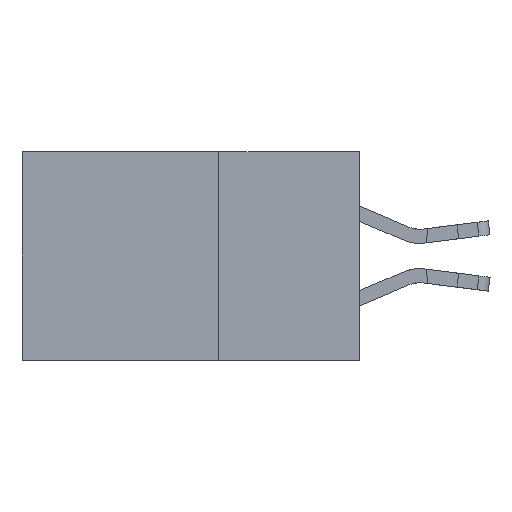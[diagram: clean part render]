
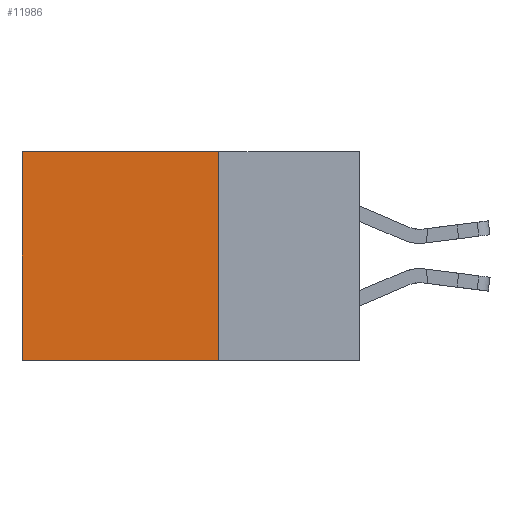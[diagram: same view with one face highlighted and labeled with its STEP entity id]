
A CAD part, left-side view. The second image highlights one B-rep face of the part: STEP entity #11986.
In plain terms, the highlighted planar face has unit normal (-1, 0, 0).
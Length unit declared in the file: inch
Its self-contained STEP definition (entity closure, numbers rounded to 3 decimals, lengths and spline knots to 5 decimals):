
#1357 = CARTESIAN_POINT ( 'NONE',  ( 0.2875, 0.6, 0. ) ) ;
#1444 = AXIS2_PLACEMENT_3D ( 'NONE', #11894, #2779, #13397 ) ;
#1705 = EDGE_CURVE ( 'NONE', #4760, #7678, #9767, .T. ) ;
#1989 = VECTOR ( 'NONE', #11844, 39.37008 ) ;
#2409 = ORIENTED_EDGE ( 'NONE', *, *, #8703, .F. ) ;
#2779 = DIRECTION ( 'NONE',  ( 1., 0., 0. ) ) ;
#3155 = CARTESIAN_POINT ( 'NONE',  ( 0.2875, 0.25, 0. ) ) ;
#3195 = VERTEX_POINT ( 'NONE', #11179 ) ;
#3923 = VECTOR ( 'NONE', #14336, 39.37008 ) ;
#4669 = VECTOR ( 'NONE', #4840, 39.37008 ) ;
#4675 = EDGE_CURVE ( 'NONE', #18759, #3195, #18023, .T. ) ;
#4760 = VERTEX_POINT ( 'NONE', #9041 ) ;
#4840 = DIRECTION ( 'NONE',  ( 0., 1., 0. ) ) ;
#6440 = CARTESIAN_POINT ( 'NONE',  ( 0.2875, 0.25, -0.37 ) ) ;
#6936 = ORIENTED_EDGE ( 'NONE', *, *, #4675, .F. ) ;
#7443 = ORIENTED_EDGE ( 'NONE', *, *, #10565, .T. ) ;
#7678 = VERTEX_POINT ( 'NONE', #17690 ) ;
#8703 = EDGE_CURVE ( 'NONE', #3195, #7678, #8784, .T. ) ;
#8784 = LINE ( 'NONE', #6440, #4669 ) ;
#9041 = CARTESIAN_POINT ( 'NONE',  ( 0.2875, 0.6, 0. ) ) ;
#9308 = VECTOR ( 'NONE', #10592, 39.37008 ) ;
#9767 = LINE ( 'NONE', #1357, #9308 ) ;
#10351 = CARTESIAN_POINT ( 'NONE',  ( 0.2875, 0.25, 0. ) ) ;
#10565 = EDGE_CURVE ( 'NONE', #18759, #4760, #15951, .T. ) ;
#10592 = DIRECTION ( 'NONE',  ( 0., 0., -1. ) ) ;
#11179 = CARTESIAN_POINT ( 'NONE',  ( 0.2875, 0.25, -0.37 ) ) ;
#11844 = DIRECTION ( 'NONE',  ( 0., 0., -1. ) ) ;
#11894 = CARTESIAN_POINT ( 'NONE',  ( 0.2875, 0.25, 0. ) ) ;
#11986 = ADVANCED_FACE ( 'NONE', ( #15643 ), #19264, .F. ) ;
#13397 = DIRECTION ( 'NONE',  ( 0., 0., -1. ) ) ;
#13584 = ORIENTED_EDGE ( 'NONE', *, *, #1705, .T. ) ;
#14336 = DIRECTION ( 'NONE',  ( 0., 1., 0. ) ) ;
#14966 = EDGE_LOOP ( 'NONE', ( #13584, #2409, #6936, #7443 ) ) ;
#15643 = FACE_OUTER_BOUND ( 'NONE', #14966, .T. ) ;
#15951 = LINE ( 'NONE', #17366, #3923 ) ;
#17366 = CARTESIAN_POINT ( 'NONE',  ( 0.2875, 0.25, 0. ) ) ;
#17690 = CARTESIAN_POINT ( 'NONE',  ( 0.2875, 0.6, -0.37 ) ) ;
#18023 = LINE ( 'NONE', #10351, #1989 ) ;
#18759 = VERTEX_POINT ( 'NONE', #3155 ) ;
#19264 = PLANE ( 'NONE',  #1444 ) ;
